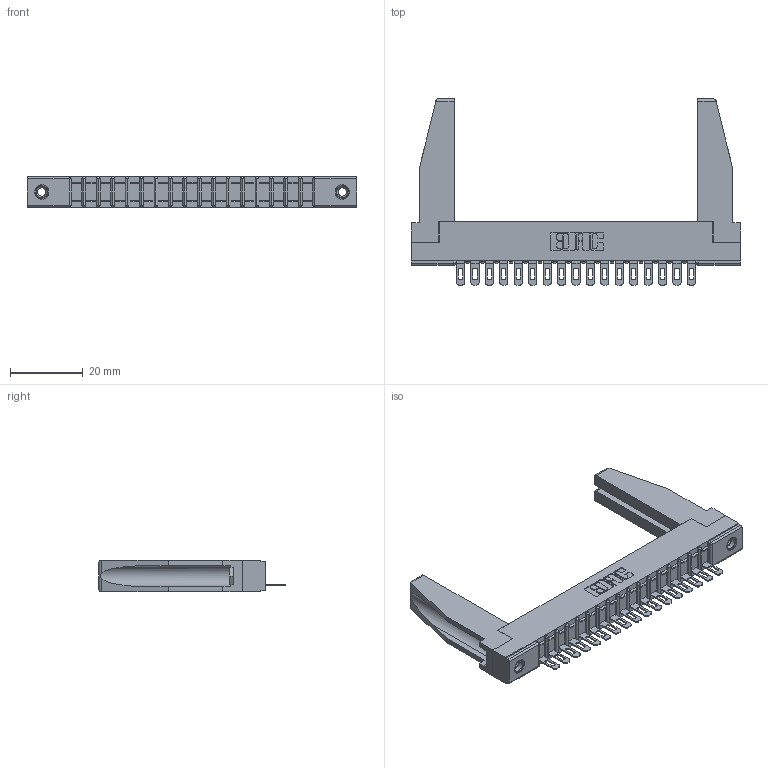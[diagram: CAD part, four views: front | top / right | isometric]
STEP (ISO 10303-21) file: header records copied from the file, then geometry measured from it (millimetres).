
FILE_DESCRIPTION (( 'STEP AP203' ), '1' );
FILE_NAME ('357-017-401-178.STEP', '2020-09-30T22:36:59', ( '' ), ( '' ), 'SwSTEP 2.0', 'SolidWorks 2020', '' );
FILE_SCHEMA (( 'CONFIG_CONTROL_DESIGN' ));
Length unit declared in the file: inch
Products named in the file (5): 357-017-401-178; 345-250-001_345-250-001-102; 307 Part_.156 Dia Mounting Holes; 307-290-002_501; 307-220-078
Assembly tree (22 placements, depth 2):
  357-017-401-178
    307 Part_.156 Dia Mounting Holes
    307-290-002_501  x17
    307-220-078  x2
    345-250-001_345-250-001-102  x2
Bounding box: 90.37 x 51.13 x 8.71 mm (x, y, z)
Volume: 9971.8 mm3; surface area: 14531 mm2
Topology: 22 solids, 22 shells, 1558 faces, 4699 edges, 3074 vertices
Faces by surface type: plane 902, cylinder 604, sphere 36, cone 12, torus 4
Entity records: 20889 total; most frequent: CARTESIAN_POINT 3518, ORIENTED_EDGE 3464, DIRECTION 3390, EDGE_CURVE 1732, LINE 1314, VECTOR 1314, VERTEX_POINT 1124, AXIS2_PLACEMENT_3D 1038
